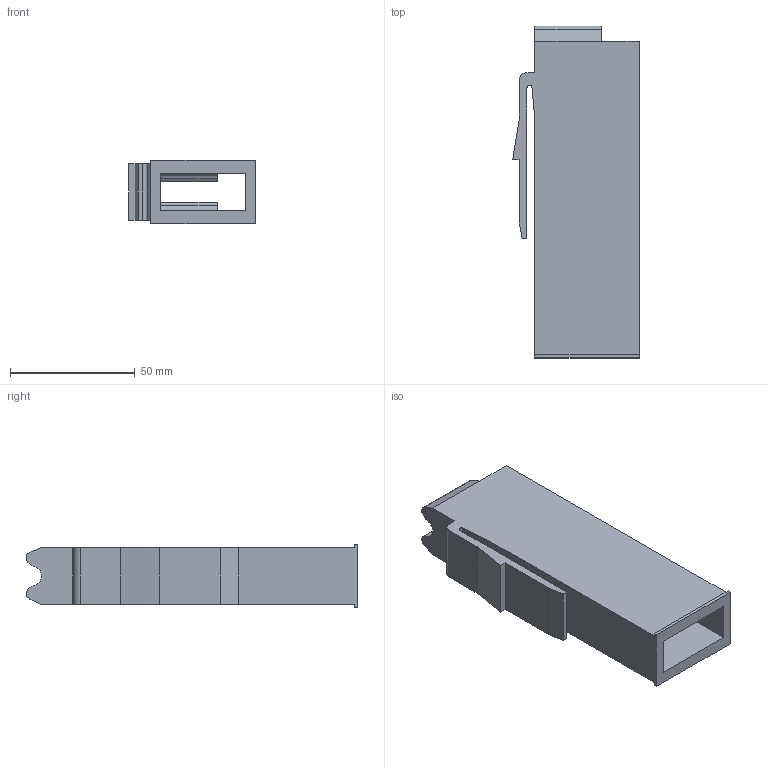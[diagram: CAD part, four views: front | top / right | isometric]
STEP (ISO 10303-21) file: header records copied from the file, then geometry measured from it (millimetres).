
FILE_DESCRIPTION (( 'STEP AP214' ), '1' );
FILE_NAME ('mag.STEP', '2013-11-06T01:47:14', ( '' ), ( '' ), 'SwSTEP 2.0', 'SolidWorks 2013', '' );
FILE_SCHEMA (( 'AUTOMOTIVE_DESIGN' ));
Length unit declared in the file: inch
Products named in the file (1): mag
Bounding box: 50.8 x 133.16 x 25.4 mm (x, y, z)
Volume: 62588.5 mm3; surface area: 34517.4 mm2
Topology: 1 solids, 1 shells, 41 faces, 114 edges, 74 vertices
Faces by surface type: plane 32, cylinder 9
Entity records: 1342 total; most frequent: CARTESIAN_POINT 230, ORIENTED_EDGE 228, DIRECTION 216, EDGE_CURVE 114, VECTOR 96, LINE 96, VERTEX_POINT 74, AXIS2_PLACEMENT_3D 60
